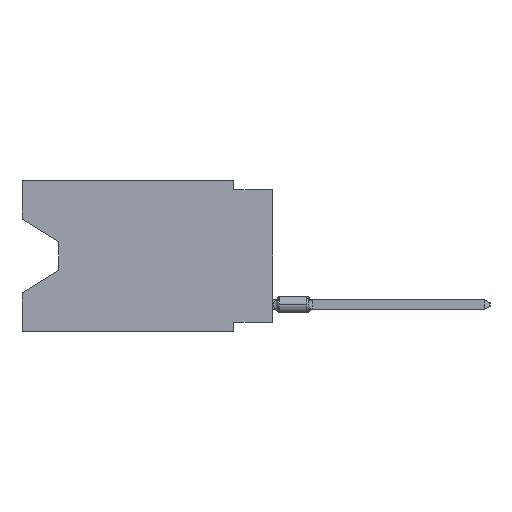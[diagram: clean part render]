
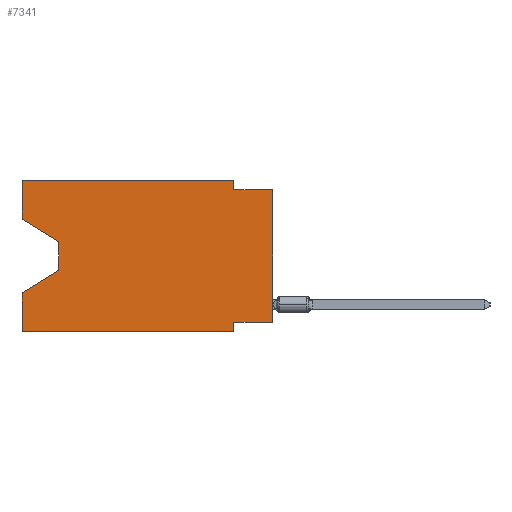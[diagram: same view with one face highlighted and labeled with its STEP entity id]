
A CAD part, left-side view. The second image highlights one B-rep face of the part: STEP entity #7341.
In plain terms, the highlighted planar face has unit normal (-1, 0, 0).
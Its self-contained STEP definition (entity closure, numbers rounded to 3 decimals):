
#413 = ORIENTED_EDGE ( 'NONE', *, *, #32334, .F. ) ;
#758 = DIRECTION ( 'NONE',  ( 0., 0., -1. ) ) ;
#1030 = FACE_OUTER_BOUND ( 'NONE', #49413, .T. ) ;
#1127 = EDGE_CURVE ( 'NONE', #26280, #28667, #30762, .T. ) ;
#1325 = VECTOR ( 'NONE', #13399, 1000. ) ;
#2210 = LINE ( 'NONE', #23358, #52081 ) ;
#2367 = ORIENTED_EDGE ( 'NONE', *, *, #17121, .T. ) ;
#3283 = CARTESIAN_POINT ( 'NONE',  ( 0., 16.383, -9.906 ) ) ;
#3350 = EDGE_CURVE ( 'NONE', #37079, #31538, #19181, .T. ) ;
#3453 = CARTESIAN_POINT ( 'NONE',  ( 0., 2.54, 0. ) ) ;
#4251 = VERTEX_POINT ( 'NONE', #46441 ) ;
#4672 = VECTOR ( 'NONE', #30346, 1000. ) ;
#4937 = VECTOR ( 'NONE', #38281, 1000. ) ;
#5117 = DIRECTION ( 'NONE',  ( 0., 0., -1. ) ) ;
#7341 = ADVANCED_FACE ( 'NONE', ( #1030 ), #36834, .F. ) ;
#7598 = DIRECTION ( 'NONE',  ( 0., 0., 1. ) ) ;
#9786 = DIRECTION ( 'NONE',  ( 0., 0., -1. ) ) ;
#12121 = ORIENTED_EDGE ( 'NONE', *, *, #14284, .F. ) ;
#12435 = LINE ( 'NONE', #44989, #4672 ) ;
#12518 = DIRECTION ( 'NONE',  ( 0., 1., 0. ) ) ;
#12755 = CARTESIAN_POINT ( 'NONE',  ( 0., 2.54, -9.271 ) ) ;
#13399 = DIRECTION ( 'NONE',  ( 0., 0.855, -0.519 ) ) ;
#13664 = LINE ( 'NONE', #54438, #24452 ) ;
#14284 = EDGE_CURVE ( 'NONE', #49574, #14718, #20351, .T. ) ;
#14718 = VERTEX_POINT ( 'NONE', #53390 ) ;
#14773 = VECTOR ( 'NONE', #28592, 1000. ) ;
#15102 = CARTESIAN_POINT ( 'NONE',  ( 0., 13.97, -4.013 ) ) ;
#15675 = ORIENTED_EDGE ( 'NONE', *, *, #3350, .F. ) ;
#17115 = AXIS2_PLACEMENT_3D ( 'NONE', #26869, #18613, #5117 ) ;
#17121 = EDGE_CURVE ( 'NONE', #42804, #14718, #51933, .T. ) ;
#18613 = DIRECTION ( 'NONE',  ( 1., 0., 0. ) ) ;
#19075 = ORIENTED_EDGE ( 'NONE', *, *, #51640, .T. ) ;
#19181 = LINE ( 'NONE', #32102, #35652 ) ;
#20058 = LINE ( 'NONE', #28873, #14773 ) ;
#20099 = DIRECTION ( 'NONE',  ( 0., -1., 0. ) ) ;
#20262 = ORIENTED_EDGE ( 'NONE', *, *, #1127, .F. ) ;
#20281 = VERTEX_POINT ( 'NONE', #12755 ) ;
#20351 = LINE ( 'NONE', #47352, #4937 ) ;
#22235 = VERTEX_POINT ( 'NONE', #35038 ) ;
#22389 = ORIENTED_EDGE ( 'NONE', *, *, #45360, .T. ) ;
#23358 = CARTESIAN_POINT ( 'NONE',  ( 0., 0., -0.635 ) ) ;
#24452 = VECTOR ( 'NONE', #758, 1000. ) ;
#24709 = VECTOR ( 'NONE', #12518, 1000. ) ;
#26082 = CARTESIAN_POINT ( 'NONE',  ( 0., 0., -9.271 ) ) ;
#26280 = VERTEX_POINT ( 'NONE', #36088 ) ;
#26869 = CARTESIAN_POINT ( 'NONE',  ( 0., 16.383, 0. ) ) ;
#27295 = VECTOR ( 'NONE', #42579, 1000. ) ;
#28592 = DIRECTION ( 'NONE',  ( 0., -1., 0. ) ) ;
#28667 = VERTEX_POINT ( 'NONE', #38404 ) ;
#28873 = CARTESIAN_POINT ( 'NONE',  ( 0., 16.383, 0. ) ) ;
#29259 = LINE ( 'NONE', #48299, #24709 ) ;
#30346 = DIRECTION ( 'NONE',  ( 0., -1., 0. ) ) ;
#30762 = LINE ( 'NONE', #57462, #43756 ) ;
#31538 = VERTEX_POINT ( 'NONE', #55184 ) ;
#32102 = CARTESIAN_POINT ( 'NONE',  ( 0., 2.54, 0. ) ) ;
#32334 = EDGE_CURVE ( 'NONE', #28667, #37079, #20058, .T. ) ;
#32615 = LINE ( 'NONE', #46961, #27295 ) ;
#33443 = CARTESIAN_POINT ( 'NONE',  ( 0., 16.383, -2.546 ) ) ;
#35038 = CARTESIAN_POINT ( 'NONE',  ( 0., 2.54, -9.906 ) ) ;
#35652 = VECTOR ( 'NONE', #9786, 1000. ) ;
#35859 = EDGE_CURVE ( 'NONE', #20281, #22235, #13664, .T. ) ;
#36088 = CARTESIAN_POINT ( 'NONE',  ( 0., 16.383, -2.546 ) ) ;
#36172 = VERTEX_POINT ( 'NONE', #52642 ) ;
#36834 = PLANE ( 'NONE',  #17115 ) ;
#37079 = VERTEX_POINT ( 'NONE', #3453 ) ;
#38143 = EDGE_CURVE ( 'NONE', #46287, #4251, #32615, .T. ) ;
#38281 = DIRECTION ( 'NONE',  ( 0., 0., 1. ) ) ;
#38404 = CARTESIAN_POINT ( 'NONE',  ( 0., 16.383, 0. ) ) ;
#39854 = EDGE_CURVE ( 'NONE', #31538, #4251, #2210, .T. ) ;
#40066 = ORIENTED_EDGE ( 'NONE', *, *, #48842, .F. ) ;
#42579 = DIRECTION ( 'NONE',  ( 0., 0., 1. ) ) ;
#42804 = VERTEX_POINT ( 'NONE', #57038 ) ;
#43200 = ORIENTED_EDGE ( 'NONE', *, *, #38143, .T. ) ;
#43756 = VECTOR ( 'NONE', #7598, 1000. ) ;
#44063 = VECTOR ( 'NONE', #47218, 1000. ) ;
#44519 = CARTESIAN_POINT ( 'NONE',  ( 0., 13.97, -5.893 ) ) ;
#44989 = CARTESIAN_POINT ( 'NONE',  ( 0., 16.383, -9.906 ) ) ;
#45360 = EDGE_CURVE ( 'NONE', #26280, #36172, #46919, .T. ) ;
#45432 = ORIENTED_EDGE ( 'NONE', *, *, #53401, .T. ) ;
#46287 = VERTEX_POINT ( 'NONE', #26082 ) ;
#46441 = CARTESIAN_POINT ( 'NONE',  ( 0., 0., -0.635 ) ) ;
#46494 = DIRECTION ( 'NONE',  ( 0., 0., -1. ) ) ;
#46919 = LINE ( 'NONE', #33443, #44063 ) ;
#46961 = CARTESIAN_POINT ( 'NONE',  ( 0., 0., 0. ) ) ;
#47218 = DIRECTION ( 'NONE',  ( 0., -0.855, -0.519 ) ) ;
#47352 = CARTESIAN_POINT ( 'NONE',  ( 0., 16.383, 0. ) ) ;
#48299 = CARTESIAN_POINT ( 'NONE',  ( 0., 0., -9.271 ) ) ;
#48766 = ORIENTED_EDGE ( 'NONE', *, *, #39854, .F. ) ;
#48842 = EDGE_CURVE ( 'NONE', #46287, #20281, #29259, .T. ) ;
#49413 = EDGE_LOOP ( 'NONE', ( #22389, #19075, #2367, #12121, #45432, #52035, #40066, #43200, #48766, #15675, #413, #20262 ) ) ;
#49574 = VERTEX_POINT ( 'NONE', #3283 ) ;
#51640 = EDGE_CURVE ( 'NONE', #36172, #42804, #54726, .T. ) ;
#51933 = LINE ( 'NONE', #44519, #1325 ) ;
#52035 = ORIENTED_EDGE ( 'NONE', *, *, #35859, .F. ) ;
#52081 = VECTOR ( 'NONE', #20099, 1000. ) ;
#52642 = CARTESIAN_POINT ( 'NONE',  ( 0., 13.97, -4.013 ) ) ;
#53390 = CARTESIAN_POINT ( 'NONE',  ( 0., 16.383, -7.36 ) ) ;
#53401 = EDGE_CURVE ( 'NONE', #49574, #22235, #12435, .T. ) ;
#54438 = CARTESIAN_POINT ( 'NONE',  ( 0., 2.54, -9.906 ) ) ;
#54726 = LINE ( 'NONE', #15102, #56658 ) ;
#55184 = CARTESIAN_POINT ( 'NONE',  ( 0., 2.54, -0.635 ) ) ;
#56658 = VECTOR ( 'NONE', #46494, 1000. ) ;
#57038 = CARTESIAN_POINT ( 'NONE',  ( 0., 13.97, -5.893 ) ) ;
#57462 = CARTESIAN_POINT ( 'NONE',  ( 0., 16.383, 0. ) ) ;
